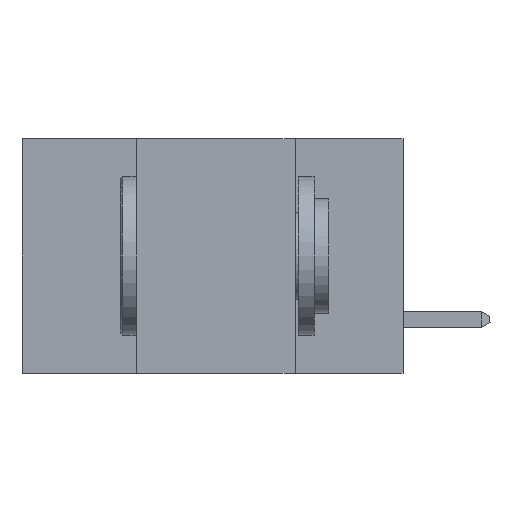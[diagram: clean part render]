
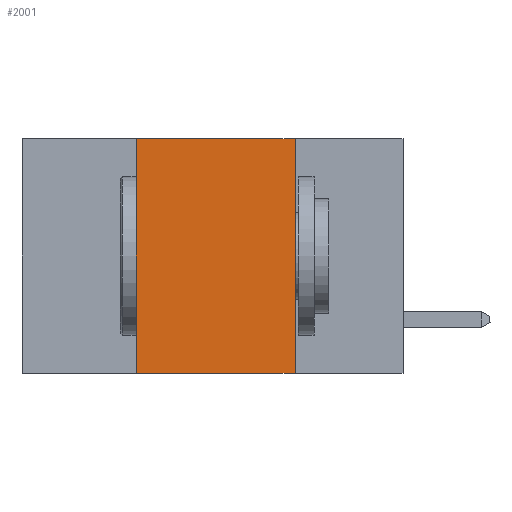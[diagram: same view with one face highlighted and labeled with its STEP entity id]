
A CAD part, left-side view. The second image highlights one B-rep face of the part: STEP entity #2001.
In plain terms, the highlighted planar face has unit normal (-1, 0, 0).
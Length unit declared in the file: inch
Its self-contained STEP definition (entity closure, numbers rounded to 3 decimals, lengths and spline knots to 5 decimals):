
#330 = AXIS2_PLACEMENT_3D ( 'NONE', #11660, #11650, #11634 ) ;
#493 = EDGE_CURVE ( 'NONE', #4607, #3997, #6127, .T. ) ;
#1079 = DIRECTION ( 'NONE',  ( 0., 0., -1. ) ) ;
#1964 = DIRECTION ( 'NONE',  ( 0., -1., 0. ) ) ;
#2001 = ADVANCED_FACE ( 'NONE', ( #4383 ), #11710, .F. ) ;
#2336 = VECTOR ( 'NONE', #2910, 39.37008 ) ;
#2341 = VECTOR ( 'NONE', #9529, 39.37008 ) ;
#2489 = VERTEX_POINT ( 'NONE', #7593 ) ;
#2910 = DIRECTION ( 'NONE',  ( 0., -1., 0. ) ) ;
#3192 = ORIENTED_EDGE ( 'NONE', *, *, #12430, .F. ) ;
#3524 = VECTOR ( 'NONE', #1079, 39.37008 ) ;
#3656 = CARTESIAN_POINT ( 'NONE',  ( 0., 0.17, 0. ) ) ;
#3919 = ORIENTED_EDGE ( 'NONE', *, *, #11209, .T. ) ;
#3927 = CARTESIAN_POINT ( 'NONE',  ( 0., 0.42, 0. ) ) ;
#3997 = VERTEX_POINT ( 'NONE', #9355 ) ;
#4383 = FACE_OUTER_BOUND ( 'NONE', #10730, .T. ) ;
#4607 = VERTEX_POINT ( 'NONE', #5584 ) ;
#4756 = CARTESIAN_POINT ( 'NONE',  ( 0., 0.42, 0. ) ) ;
#4807 = LINE ( 'NONE', #11491, #12044 ) ;
#5584 = CARTESIAN_POINT ( 'NONE',  ( 0., 0.17, 0. ) ) ;
#6037 = ORIENTED_EDGE ( 'NONE', *, *, #6739, .F. ) ;
#6127 = LINE ( 'NONE', #3656, #3524 ) ;
#6163 = VERTEX_POINT ( 'NONE', #3927 ) ;
#6739 = EDGE_CURVE ( 'NONE', #6163, #4607, #9968, .T. ) ;
#7204 = LINE ( 'NONE', #4756, #2341 ) ;
#7593 = CARTESIAN_POINT ( 'NONE',  ( 0., 0.42, -0.37 ) ) ;
#9355 = CARTESIAN_POINT ( 'NONE',  ( 0., 0.17, -0.37 ) ) ;
#9529 = DIRECTION ( 'NONE',  ( 0., 0., 1. ) ) ;
#9968 = LINE ( 'NONE', #10509, #2336 ) ;
#10209 = ORIENTED_EDGE ( 'NONE', *, *, #493, .F. ) ;
#10509 = CARTESIAN_POINT ( 'NONE',  ( 0., 0.6, 0. ) ) ;
#10730 = EDGE_LOOP ( 'NONE', ( #10209, #6037, #3192, #3919 ) ) ;
#11209 = EDGE_CURVE ( 'NONE', #2489, #3997, #4807, .T. ) ;
#11491 = CARTESIAN_POINT ( 'NONE',  ( 0., 0.6, -0.37 ) ) ;
#11634 = DIRECTION ( 'NONE',  ( 0., 0., -1. ) ) ;
#11650 = DIRECTION ( 'NONE',  ( 1., 0., 0. ) ) ;
#11660 = CARTESIAN_POINT ( 'NONE',  ( 0., 0.6, 0. ) ) ;
#11710 = PLANE ( 'NONE',  #330 ) ;
#12044 = VECTOR ( 'NONE', #1964, 39.37008 ) ;
#12430 = EDGE_CURVE ( 'NONE', #2489, #6163, #7204, .T. ) ;
